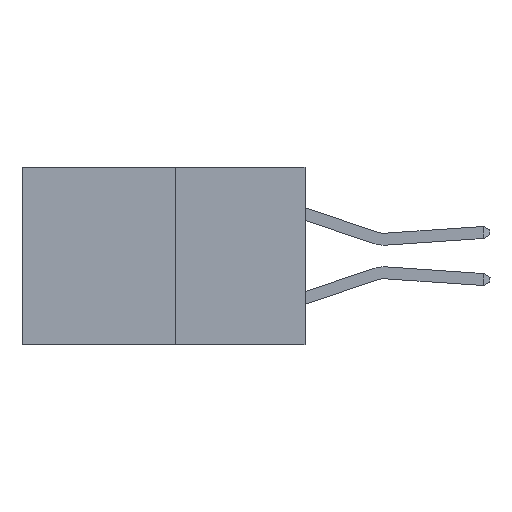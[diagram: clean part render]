
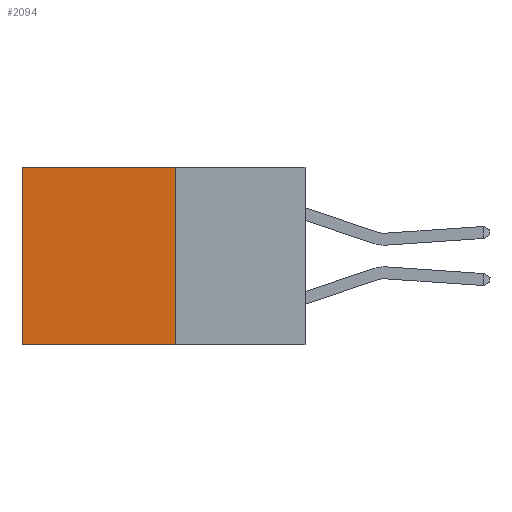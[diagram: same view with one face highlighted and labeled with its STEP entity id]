
A CAD part, left-side view. The second image highlights one B-rep face of the part: STEP entity #2094.
In plain terms, the highlighted planar face has unit normal (-1, 0, 0).
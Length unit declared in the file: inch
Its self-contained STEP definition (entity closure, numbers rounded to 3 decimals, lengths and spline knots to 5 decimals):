
#114 = DIRECTION ( 'NONE',  ( 0., 0., -1. ) ) ;
#306 = LINE ( 'NONE', #8474, #8462 ) ;
#363 = CARTESIAN_POINT ( 'NONE',  ( 0.277, 0.27, -0.37 ) ) ;
#369 = DIRECTION ( 'NONE',  ( 0., 0., -1. ) ) ;
#534 = ORIENTED_EDGE ( 'NONE', *, *, #6640, .F. ) ;
#659 = VERTEX_POINT ( 'NONE', #8298 ) ;
#669 = VERTEX_POINT ( 'NONE', #7649 ) ;
#786 = CARTESIAN_POINT ( 'NONE',  ( 0.277, 0.27, 0. ) ) ;
#909 = CARTESIAN_POINT ( 'NONE',  ( 0.277, 0.59, -0.37 ) ) ;
#1540 = EDGE_CURVE ( 'NONE', #8835, #659, #7150, .T. ) ;
#2094 = ADVANCED_FACE ( 'NONE', ( #7704 ), #6912, .F. ) ;
#2849 = ORIENTED_EDGE ( 'NONE', *, *, #3432, .T. ) ;
#3037 = VECTOR ( 'NONE', #6269, 39.37008 ) ;
#3432 = EDGE_CURVE ( 'NONE', #7939, #8835, #8427, .T. ) ;
#4185 = LINE ( 'NONE', #6128, #4440 ) ;
#4359 = AXIS2_PLACEMENT_3D ( 'NONE', #363, #9939, #114 ) ;
#4440 = VECTOR ( 'NONE', #369, 39.37008 ) ;
#4792 = DIRECTION ( 'NONE',  ( 0., 1., 0. ) ) ;
#5198 = ORIENTED_EDGE ( 'NONE', *, *, #9966, .F. ) ;
#6128 = CARTESIAN_POINT ( 'NONE',  ( 0.277, 0.27, -0.37 ) ) ;
#6269 = DIRECTION ( 'NONE',  ( 0., 0., -1. ) ) ;
#6294 = VECTOR ( 'NONE', #4792, 39.37008 ) ;
#6640 = EDGE_CURVE ( 'NONE', #7939, #669, #4185, .T. ) ;
#6912 = PLANE ( 'NONE',  #4359 ) ;
#7150 = LINE ( 'NONE', #909, #3037 ) ;
#7320 = EDGE_LOOP ( 'NONE', ( #8847, #5198, #534, #2849 ) ) ;
#7398 = CARTESIAN_POINT ( 'NONE',  ( 0.277, 0.27, 0. ) ) ;
#7649 = CARTESIAN_POINT ( 'NONE',  ( 0.277, 0.27, -0.37 ) ) ;
#7704 = FACE_OUTER_BOUND ( 'NONE', #7320, .T. ) ;
#7939 = VERTEX_POINT ( 'NONE', #7398 ) ;
#8298 = CARTESIAN_POINT ( 'NONE',  ( 0.277, 0.59, -0.37 ) ) ;
#8427 = LINE ( 'NONE', #786, #6294 ) ;
#8462 = VECTOR ( 'NONE', #9190, 39.37008 ) ;
#8474 = CARTESIAN_POINT ( 'NONE',  ( 0.277, 0.27, -0.37 ) ) ;
#8835 = VERTEX_POINT ( 'NONE', #9039 ) ;
#8847 = ORIENTED_EDGE ( 'NONE', *, *, #1540, .T. ) ;
#9039 = CARTESIAN_POINT ( 'NONE',  ( 0.277, 0.59, 0. ) ) ;
#9190 = DIRECTION ( 'NONE',  ( 0., 1., 0. ) ) ;
#9939 = DIRECTION ( 'NONE',  ( 1., 0., 0. ) ) ;
#9966 = EDGE_CURVE ( 'NONE', #669, #659, #306, .T. ) ;
